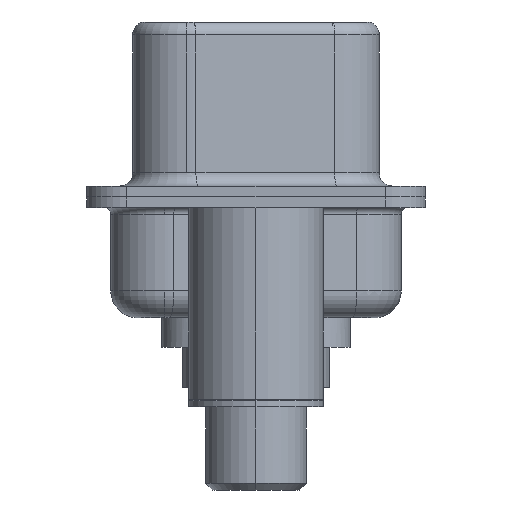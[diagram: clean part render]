
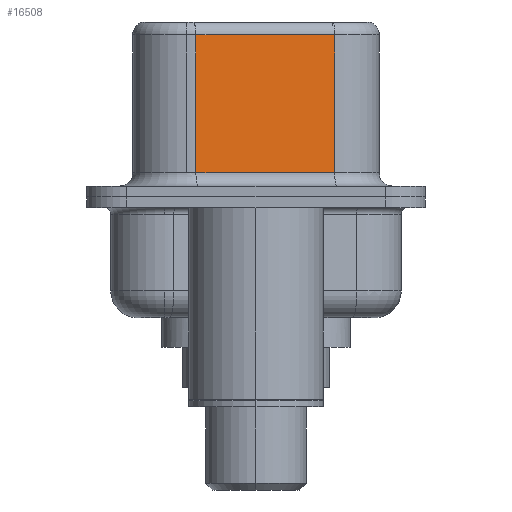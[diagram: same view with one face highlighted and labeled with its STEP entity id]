
A CAD part, left-side view. The second image highlights one B-rep face of the part: STEP entity #16508.
In plain terms, the highlighted planar face has unit normal (-0.985, -0.174, 0).
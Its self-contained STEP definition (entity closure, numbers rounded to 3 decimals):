
#1871 = CARTESIAN_POINT ( 'NONE',  ( 3.67, 2.233, 6.02 ) ) ;
#1981 = ORIENTED_EDGE ( 'NONE', *, *, #12514, .T. ) ;
#2157 = ORIENTED_EDGE ( 'NONE', *, *, #5492, .T. ) ;
#2491 = ORIENTED_EDGE ( 'NONE', *, *, #10910, .T. ) ;
#4503 = CARTESIAN_POINT ( 'NONE',  ( 4.58, -2.927, 6.02 ) ) ;
#4580 = VERTEX_POINT ( 'NONE', #18599 ) ;
#4742 = DIRECTION ( 'NONE',  ( 0.985, 0.174, 0. ) ) ;
#5249 = VERTEX_POINT ( 'NONE', #1871 ) ;
#5492 = EDGE_CURVE ( 'NONE', #6953, #5249, #16334, .T. ) ;
#6409 = VECTOR ( 'NONE', #14720, 1000. ) ;
#6788 = VECTOR ( 'NONE', #8494, 1000. ) ;
#6953 = VERTEX_POINT ( 'NONE', #12091 ) ;
#7687 = EDGE_CURVE ( 'NONE', #6953, #4580, #15264, .T. ) ;
#8274 = CARTESIAN_POINT ( 'NONE',  ( 4.58, -2.927, 0.9 ) ) ;
#8494 = DIRECTION ( 'NONE',  ( 0.174, -0.985, 0. ) ) ;
#9473 = DIRECTION ( 'NONE',  ( -0.174, 0.985, 0. ) ) ;
#10475 = LINE ( 'NONE', #8274, #6788 ) ;
#10910 = EDGE_CURVE ( 'NONE', #18374, #4580, #10475, .T. ) ;
#12091 = CARTESIAN_POINT ( 'NONE',  ( 4.58, -2.927, 6.02 ) ) ;
#12514 = EDGE_CURVE ( 'NONE', #5249, #18374, #14787, .T. ) ;
#12545 = VECTOR ( 'NONE', #15700, 1000. ) ;
#12658 = CARTESIAN_POINT ( 'NONE',  ( 4.58, -2.927, 6.52 ) ) ;
#13898 = DIRECTION ( 'NONE',  ( -0.174, 0.985, 0. ) ) ;
#14720 = DIRECTION ( 'NONE',  ( 0., 0., -1. ) ) ;
#14787 = LINE ( 'NONE', #19543, #6409 ) ;
#15166 = FACE_OUTER_BOUND ( 'NONE', #16026, .T. ) ;
#15264 = LINE ( 'NONE', #12658, #12545 ) ;
#15700 = DIRECTION ( 'NONE',  ( 0., 0., -1. ) ) ;
#16026 = EDGE_LOOP ( 'NONE', ( #20076, #2157, #1981, #2491 ) ) ;
#16334 = LINE ( 'NONE', #4503, #17809 ) ;
#16508 = ADVANCED_FACE ( 'NONE', ( #15166 ), #17462, .F. ) ;
#17133 = CARTESIAN_POINT ( 'NONE',  ( 3.67, 2.233, 0.9 ) ) ;
#17462 = PLANE ( 'NONE',  #18089 ) ;
#17809 = VECTOR ( 'NONE', #13898, 1000. ) ;
#18089 = AXIS2_PLACEMENT_3D ( 'NONE', #19094, #4742, #9473 ) ;
#18374 = VERTEX_POINT ( 'NONE', #17133 ) ;
#18599 = CARTESIAN_POINT ( 'NONE',  ( 4.58, -2.927, 0.9 ) ) ;
#19094 = CARTESIAN_POINT ( 'NONE',  ( 4.58, -2.927, 6.52 ) ) ;
#19543 = CARTESIAN_POINT ( 'NONE',  ( 3.67, 2.233, 6.52 ) ) ;
#20076 = ORIENTED_EDGE ( 'NONE', *, *, #7687, .F. ) ;
